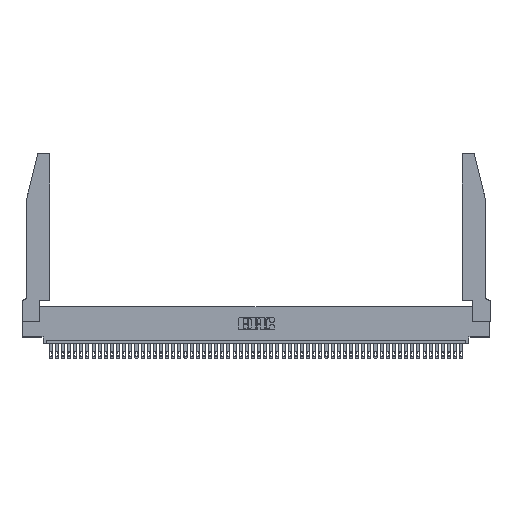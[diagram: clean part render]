
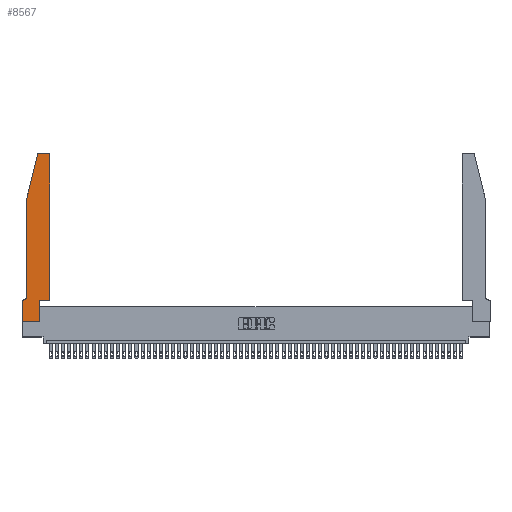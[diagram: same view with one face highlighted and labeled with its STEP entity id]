
A CAD part, top view. The second image highlights one B-rep face of the part: STEP entity #8567.
In plain terms, the highlighted planar face has unit normal (0, 0, 1).
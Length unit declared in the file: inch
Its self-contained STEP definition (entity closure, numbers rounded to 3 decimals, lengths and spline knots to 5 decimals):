
#1054 = CARTESIAN_POINT ( 'NONE',  ( 0.4505, 2.72, 0.37 ) ) ;
#1465 = CARTESIAN_POINT ( 'NONE',  ( 0.0755, 0.42, 0.37 ) ) ;
#1902 = AXIS2_PLACEMENT_3D ( 'NONE', #10135, #5897, #15155 ) ;
#2168 = DIRECTION ( 'NONE',  ( 0., 0., -1. ) ) ;
#2695 = CARTESIAN_POINT ( 'NONE',  ( 0., 0., 0.37 ) ) ;
#3031 = CARTESIAN_POINT ( 'NONE',  ( 0.2865, 0.35, 0.37 ) ) ;
#3171 = CARTESIAN_POINT ( 'NONE',  ( 0.0755, 2., 0.37 ) ) ;
#3602 = CARTESIAN_POINT ( 'NONE',  ( 0.4505, 0.35, 0.37 ) ) ;
#3655 = PLANE ( 'NONE',  #24046 ) ;
#3973 = VECTOR ( 'NONE', #46809, 39.37008 ) ;
#4107 = LINE ( 'NONE', #3171, #47246 ) ;
#4181 = ORIENTED_EDGE ( 'NONE', *, *, #26364, .T. ) ;
#4220 = ORIENTED_EDGE ( 'NONE', *, *, #16877, .T. ) ;
#4883 = ORIENTED_EDGE ( 'NONE', *, *, #25225, .T. ) ;
#5833 = DIRECTION ( 'NONE',  ( 0., 0., 1. ) ) ;
#5897 = DIRECTION ( 'NONE',  ( 0., 0., 1. ) ) ;
#7574 = CIRCLE ( 'NONE', #20139, 0.03 ) ;
#7876 = ORIENTED_EDGE ( 'NONE', *, *, #40647, .T. ) ;
#7959 = VERTEX_POINT ( 'NONE', #3602 ) ;
#8505 = DIRECTION ( 'NONE',  ( 1., 0., 0. ) ) ;
#8567 = ADVANCED_FACE ( 'NONE', ( #47348 ), #3655, .T. ) ;
#8840 = DIRECTION ( 'NONE',  ( -1., 0., 0. ) ) ;
#9914 = CARTESIAN_POINT ( 'NONE',  ( 0.0055, 0.42, 0.37 ) ) ;
#10135 = CARTESIAN_POINT ( 'NONE',  ( 0.284, 2.72, 0.37 ) ) ;
#10441 = CIRCLE ( 'NONE', #43785, 0.07 ) ;
#11633 = DIRECTION ( 'NONE',  ( 0., -1., 0. ) ) ;
#11780 = LINE ( 'NONE', #18012, #52409 ) ;
#11838 = LINE ( 'NONE', #39674, #19458 ) ;
#12013 = LINE ( 'NONE', #48139, #29764 ) ;
#12297 = VERTEX_POINT ( 'NONE', #14427 ) ;
#12433 = VERTEX_POINT ( 'NONE', #50153 ) ;
#13704 = CARTESIAN_POINT ( 'NONE',  ( 0.25487, 2.72718, 0.37 ) ) ;
#14427 = CARTESIAN_POINT ( 'NONE',  ( 0.2865, 0.35, 0.37 ) ) ;
#14824 = VERTEX_POINT ( 'NONE', #1465 ) ;
#15155 = DIRECTION ( 'NONE',  ( 1., 0., 0. ) ) ;
#15158 = DIRECTION ( 'NONE',  ( 0., 0., 1. ) ) ;
#15395 = EDGE_CURVE ( 'NONE', #7959, #19825, #26199, .T. ) ;
#16877 = EDGE_CURVE ( 'NONE', #33480, #23381, #40349, .T. ) ;
#18012 = CARTESIAN_POINT ( 'NONE',  ( 0.0755, 2., 0.37 ) ) ;
#19458 = VECTOR ( 'NONE', #30992, 39.37008 ) ;
#19495 = ORIENTED_EDGE ( 'NONE', *, *, #29269, .T. ) ;
#19611 = ORIENTED_EDGE ( 'NONE', *, *, #25882, .T. ) ;
#19825 = VERTEX_POINT ( 'NONE', #1054 ) ;
#20139 = AXIS2_PLACEMENT_3D ( 'NONE', #43308, #5833, #51678 ) ;
#20437 = VECTOR ( 'NONE', #50338, 39.37008 ) ;
#21351 = VERTEX_POINT ( 'NONE', #13704 ) ;
#21672 = CARTESIAN_POINT ( 'NONE',  ( 0., 0., 0.37 ) ) ;
#22093 = DIRECTION ( 'NONE',  ( -0.239, -0.971, 0. ) ) ;
#22923 = EDGE_CURVE ( 'NONE', #21351, #27731, #11780, .T. ) ;
#23166 = EDGE_CURVE ( 'NONE', #23381, #12297, #27483, .T. ) ;
#23311 = ORIENTED_EDGE ( 'NONE', *, *, #25382, .T. ) ;
#23381 = VERTEX_POINT ( 'NONE', #42848 ) ;
#24046 = AXIS2_PLACEMENT_3D ( 'NONE', #51689, #15158, #8505 ) ;
#24766 = CARTESIAN_POINT ( 'NONE',  ( 0.4505, 0.35, 0.37 ) ) ;
#25225 = EDGE_CURVE ( 'NONE', #12297, #7959, #11838, .T. ) ;
#25382 = EDGE_CURVE ( 'NONE', #27868, #33480, #50511, .T. ) ;
#25882 = EDGE_CURVE ( 'NONE', #36208, #21351, #51764, .T. ) ;
#26199 = LINE ( 'NONE', #24766, #20437 ) ;
#26364 = EDGE_CURVE ( 'NONE', #14824, #50896, #10441, .T. ) ;
#26981 = CARTESIAN_POINT ( 'NONE',  ( 0.0055, 0.35, 0.37 ) ) ;
#27483 = LINE ( 'NONE', #3031, #3973 ) ;
#27533 = DIRECTION ( 'NONE',  ( 0., -1., 0. ) ) ;
#27731 = VERTEX_POINT ( 'NONE', #29538 ) ;
#27868 = VERTEX_POINT ( 'NONE', #45606 ) ;
#28490 = CARTESIAN_POINT ( 'NONE',  ( 0.284, 2.75, 0.37 ) ) ;
#29269 = EDGE_CURVE ( 'NONE', #12433, #36208, #12013, .T. ) ;
#29538 = CARTESIAN_POINT ( 'NONE',  ( 0.0755, 2., 0.37 ) ) ;
#29764 = VECTOR ( 'NONE', #44896, 39.37008 ) ;
#30992 = DIRECTION ( 'NONE',  ( 1., 0., 0. ) ) ;
#31456 = CARTESIAN_POINT ( 'NONE',  ( 0., 0., 0.37 ) ) ;
#32897 = EDGE_CURVE ( 'NONE', #27731, #14824, #4107, .T. ) ;
#33480 = VERTEX_POINT ( 'NONE', #21672 ) ;
#33569 = ORIENTED_EDGE ( 'NONE', *, *, #23166, .T. ) ;
#35406 = ORIENTED_EDGE ( 'NONE', *, *, #35725, .T. ) ;
#35725 = EDGE_CURVE ( 'NONE', #19825, #12433, #7574, .T. ) ;
#36208 = VERTEX_POINT ( 'NONE', #28490 ) ;
#36547 = LINE ( 'NONE', #41443, #39671 ) ;
#36650 = VECTOR ( 'NONE', #27533, 39.37008 ) ;
#36952 = EDGE_LOOP ( 'NONE', ( #19495, #19611, #52178, #38339, #4181, #7876, #23311, #4220, #33569, #4883, #39098, #35406 ) ) ;
#38339 = ORIENTED_EDGE ( 'NONE', *, *, #32897, .T. ) ;
#38888 = DIRECTION ( 'NONE',  ( 1., 0., 0. ) ) ;
#39098 = ORIENTED_EDGE ( 'NONE', *, *, #15395, .T. ) ;
#39671 = VECTOR ( 'NONE', #49554, 39.37008 ) ;
#39674 = CARTESIAN_POINT ( 'NONE',  ( 0.4505, 0.35, 0.37 ) ) ;
#40349 = LINE ( 'NONE', #2695, #51729 ) ;
#40647 = EDGE_CURVE ( 'NONE', #50896, #27868, #36547, .T. ) ;
#41443 = CARTESIAN_POINT ( 'NONE',  ( 0.0755, 0.35, 0.37 ) ) ;
#42848 = CARTESIAN_POINT ( 'NONE',  ( 0.2865, 0., 0.37 ) ) ;
#43308 = CARTESIAN_POINT ( 'NONE',  ( 0.4205, 2.72, 0.37 ) ) ;
#43785 = AXIS2_PLACEMENT_3D ( 'NONE', #9914, #2168, #8840 ) ;
#44896 = DIRECTION ( 'NONE',  ( -1., 0., 0. ) ) ;
#45606 = CARTESIAN_POINT ( 'NONE',  ( 0., 0.35, 0.37 ) ) ;
#46809 = DIRECTION ( 'NONE',  ( 0., 1., 0. ) ) ;
#47246 = VECTOR ( 'NONE', #11633, 39.37008 ) ;
#47348 = FACE_OUTER_BOUND ( 'NONE', #36952, .T. ) ;
#48139 = CARTESIAN_POINT ( 'NONE',  ( 0.2605, 2.75, 0.37 ) ) ;
#49554 = DIRECTION ( 'NONE',  ( -1., 0., 0. ) ) ;
#50153 = CARTESIAN_POINT ( 'NONE',  ( 0.4205, 2.75, 0.37 ) ) ;
#50338 = DIRECTION ( 'NONE',  ( 0., 1., 0. ) ) ;
#50511 = LINE ( 'NONE', #31456, #36650 ) ;
#50896 = VERTEX_POINT ( 'NONE', #26981 ) ;
#51678 = DIRECTION ( 'NONE',  ( 1., 0., 0. ) ) ;
#51689 = CARTESIAN_POINT ( 'NONE',  ( 0., 0.35, 0.37 ) ) ;
#51729 = VECTOR ( 'NONE', #38888, 39.37008 ) ;
#51764 = CIRCLE ( 'NONE', #1902, 0.03 ) ;
#52178 = ORIENTED_EDGE ( 'NONE', *, *, #22923, .T. ) ;
#52409 = VECTOR ( 'NONE', #22093, 39.37008 ) ;
